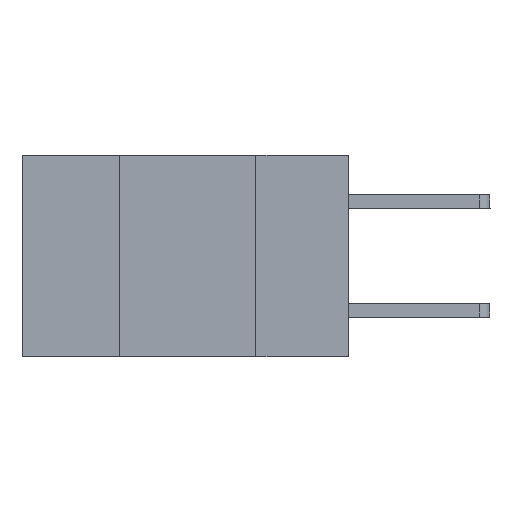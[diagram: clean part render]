
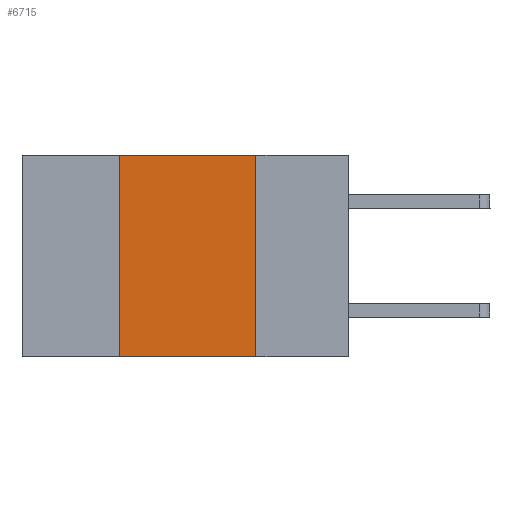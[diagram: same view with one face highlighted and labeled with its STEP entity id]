
A CAD part, left-side view. The second image highlights one B-rep face of the part: STEP entity #6715.
In plain terms, the highlighted planar face has unit normal (-1, 0, 0).
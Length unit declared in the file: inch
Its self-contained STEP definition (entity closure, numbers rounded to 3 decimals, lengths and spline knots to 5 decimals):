
#514 = LINE ( 'NONE', #4544, #4793 ) ;
#753 = VERTEX_POINT ( 'NONE', #3387 ) ;
#1312 = LINE ( 'NONE', #3223, #8483 ) ;
#1520 = CARTESIAN_POINT ( 'NONE',  ( 0., 0.6, 0. ) ) ;
#1622 = CARTESIAN_POINT ( 'NONE',  ( 0., 0.42, -0.37 ) ) ;
#1834 = VERTEX_POINT ( 'NONE', #8141 ) ;
#1880 = ORIENTED_EDGE ( 'NONE', *, *, #5889, .F. ) ;
#2443 = CARTESIAN_POINT ( 'NONE',  ( 0., 0.17, -0.37 ) ) ;
#2546 = ORIENTED_EDGE ( 'NONE', *, *, #8553, .F. ) ;
#2944 = LINE ( 'NONE', #1520, #3995 ) ;
#3223 = CARTESIAN_POINT ( 'NONE',  ( 0., 0.42, -0.37 ) ) ;
#3256 = LINE ( 'NONE', #8050, #7221 ) ;
#3387 = CARTESIAN_POINT ( 'NONE',  ( 0., 0.17, 0. ) ) ;
#3448 = ORIENTED_EDGE ( 'NONE', *, *, #3486, .F. ) ;
#3486 = EDGE_CURVE ( 'NONE', #1834, #753, #2944, .T. ) ;
#3754 = PLANE ( 'NONE',  #3876 ) ;
#3876 = AXIS2_PLACEMENT_3D ( 'NONE', #4908, #7602, #5008 ) ;
#3995 = VECTOR ( 'NONE', #6886, 39.37008 ) ;
#4033 = DIRECTION ( 'NONE',  ( 0., -1., 0. ) ) ;
#4218 = ORIENTED_EDGE ( 'NONE', *, *, #5900, .T. ) ;
#4391 = FACE_OUTER_BOUND ( 'NONE', #4574, .T. ) ;
#4544 = CARTESIAN_POINT ( 'NONE',  ( 0., 0.17, -0.37 ) ) ;
#4574 = EDGE_LOOP ( 'NONE', ( #2546, #3448, #1880, #4218 ) ) ;
#4584 = DIRECTION ( 'NONE',  ( 0., 0., -1. ) ) ;
#4793 = VECTOR ( 'NONE', #4584, 39.37008 ) ;
#4908 = CARTESIAN_POINT ( 'NONE',  ( 0., 0.6, 0. ) ) ;
#5008 = DIRECTION ( 'NONE',  ( 0., 0., -1. ) ) ;
#5672 = VERTEX_POINT ( 'NONE', #1622 ) ;
#5815 = VERTEX_POINT ( 'NONE', #2443 ) ;
#5889 = EDGE_CURVE ( 'NONE', #5672, #1834, #1312, .T. ) ;
#5900 = EDGE_CURVE ( 'NONE', #5672, #5815, #3256, .T. ) ;
#6715 = ADVANCED_FACE ( 'NONE', ( #4391 ), #3754, .F. ) ;
#6886 = DIRECTION ( 'NONE',  ( 0., -1., 0. ) ) ;
#7221 = VECTOR ( 'NONE', #4033, 39.37008 ) ;
#7602 = DIRECTION ( 'NONE',  ( 1., 0., 0. ) ) ;
#8009 = DIRECTION ( 'NONE',  ( 0., 0., 1. ) ) ;
#8050 = CARTESIAN_POINT ( 'NONE',  ( 0., 0.6, -0.37 ) ) ;
#8141 = CARTESIAN_POINT ( 'NONE',  ( 0., 0.42, 0. ) ) ;
#8483 = VECTOR ( 'NONE', #8009, 39.37008 ) ;
#8553 = EDGE_CURVE ( 'NONE', #753, #5815, #514, .T. ) ;
